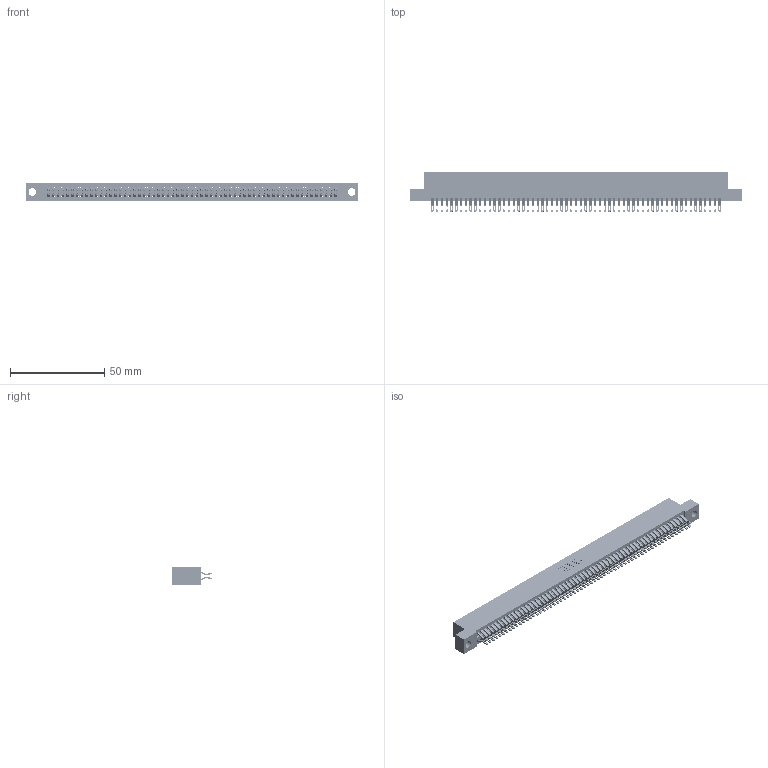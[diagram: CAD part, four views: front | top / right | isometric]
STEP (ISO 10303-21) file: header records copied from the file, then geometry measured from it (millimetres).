
FILE_DESCRIPTION (( 'STEP AP203' ), '1' );
FILE_NAME ('345-122-555-204.STEP', '2021-05-25T17:47:28', ( '' ), ( '' ), 'SwSTEP 2.0', 'SolidWorks 2020', '' );
FILE_SCHEMA (( 'CONFIG_CONTROL_DESIGN' ));
Length unit declared in the file: inch
Products named in the file (3): 345-292-001_555 Tail; 345 Part_Flush Mounting Lugs - 0.156 Dia-TI; 345-122-555-204
Assembly tree (123 placements, depth 2):
  345-122-555-204
    345 Part_Flush Mounting Lugs - 0.156 Dia-TI
    345-292-001_555 Tail  x122
Bounding box: 176.15 x 21.13 x 9.4 mm (x, y, z)
Volume: 17535.6 mm3; surface area: 27370.9 mm2
Topology: 123 solids, 123 shells, 6972 faces, 21971 edges, 14646 vertices
Faces by surface type: plane 3876, cylinder 3096
Entity records: 46049 total; most frequent: CARTESIAN_POINT 7740, ORIENTED_EDGE 7642, DIRECTION 6769, EDGE_CURVE 3821, LINE 3425, VECTOR 3425, VERTEX_POINT 2546, AXIS2_PLACEMENT_3D 1672
